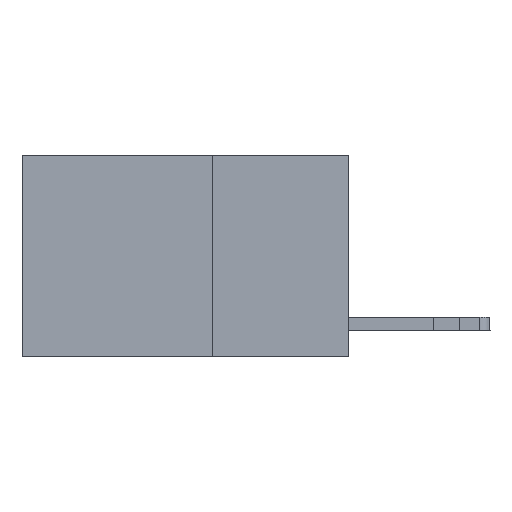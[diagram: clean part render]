
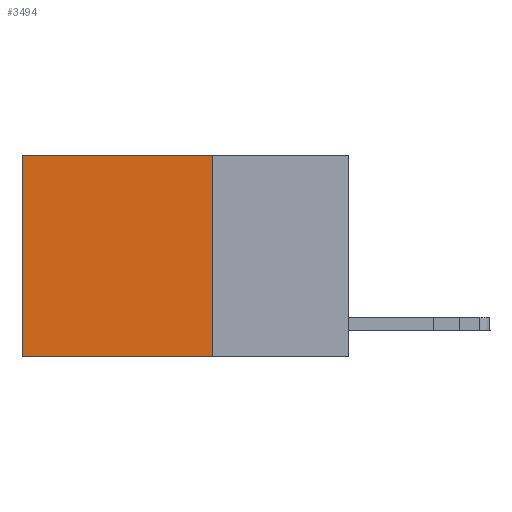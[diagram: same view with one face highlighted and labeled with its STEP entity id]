
A CAD part, left-side view. The second image highlights one B-rep face of the part: STEP entity #3494.
In plain terms, the highlighted planar face has unit normal (-1, 0, 0).
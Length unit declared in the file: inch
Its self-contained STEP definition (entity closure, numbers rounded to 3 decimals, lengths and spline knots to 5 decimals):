
#632 = ORIENTED_EDGE ( 'NONE', *, *, #12748, .T. ) ;
#1769 = VECTOR ( 'NONE', #14130, 39.37008 ) ;
#1792 = CARTESIAN_POINT ( 'NONE',  ( 0.2625, 0.25, 0. ) ) ;
#2085 = CARTESIAN_POINT ( 'NONE',  ( 0.2625, 0.25, -0.37 ) ) ;
#2788 = VECTOR ( 'NONE', #20159, 39.37008 ) ;
#2978 = VECTOR ( 'NONE', #10140, 39.37008 ) ;
#3494 = ADVANCED_FACE ( 'NONE', ( #3748 ), #18548, .F. ) ;
#3636 = LINE ( 'NONE', #5461, #2978 ) ;
#3684 = ORIENTED_EDGE ( 'NONE', *, *, #6785, .F. ) ;
#3748 = FACE_OUTER_BOUND ( 'NONE', #7550, .T. ) ;
#4170 = CARTESIAN_POINT ( 'NONE',  ( 0.2625, 0.6, 0. ) ) ;
#5211 = AXIS2_PLACEMENT_3D ( 'NONE', #11943, #18334, #7277 ) ;
#5420 = LINE ( 'NONE', #1792, #6610 ) ;
#5461 = CARTESIAN_POINT ( 'NONE',  ( 0.2625, 0.6, 0. ) ) ;
#5915 = CARTESIAN_POINT ( 'NONE',  ( 0.2625, 0.6, -0.37 ) ) ;
#6511 = ORIENTED_EDGE ( 'NONE', *, *, #18447, .T. ) ;
#6610 = VECTOR ( 'NONE', #11697, 39.37008 ) ;
#6785 = EDGE_CURVE ( 'NONE', #21086, #20830, #5420, .T. ) ;
#7277 = DIRECTION ( 'NONE',  ( 0., 0., -1. ) ) ;
#7550 = EDGE_LOOP ( 'NONE', ( #632, #9559, #3684, #6511 ) ) ;
#7853 = LINE ( 'NONE', #14338, #1769 ) ;
#9453 = VERTEX_POINT ( 'NONE', #4170 ) ;
#9559 = ORIENTED_EDGE ( 'NONE', *, *, #18653, .F. ) ;
#10140 = DIRECTION ( 'NONE',  ( 0., 0., -1. ) ) ;
#11697 = DIRECTION ( 'NONE',  ( 0., 0., -1. ) ) ;
#11943 = CARTESIAN_POINT ( 'NONE',  ( 0.2625, 0.25, 0. ) ) ;
#12748 = EDGE_CURVE ( 'NONE', #9453, #16873, #3636, .T. ) ;
#13754 = CARTESIAN_POINT ( 'NONE',  ( 0.2625, 0.25, -0.37 ) ) ;
#14130 = DIRECTION ( 'NONE',  ( 0., 1., 0. ) ) ;
#14338 = CARTESIAN_POINT ( 'NONE',  ( 0.2625, 0.25, 0. ) ) ;
#15462 = LINE ( 'NONE', #13754, #2788 ) ;
#16873 = VERTEX_POINT ( 'NONE', #5915 ) ;
#18334 = DIRECTION ( 'NONE',  ( 1., 0., 0. ) ) ;
#18447 = EDGE_CURVE ( 'NONE', #21086, #9453, #7853, .T. ) ;
#18548 = PLANE ( 'NONE',  #5211 ) ;
#18653 = EDGE_CURVE ( 'NONE', #20830, #16873, #15462, .T. ) ;
#19169 = CARTESIAN_POINT ( 'NONE',  ( 0.2625, 0.25, 0. ) ) ;
#20159 = DIRECTION ( 'NONE',  ( 0., 1., 0. ) ) ;
#20830 = VERTEX_POINT ( 'NONE', #2085 ) ;
#21086 = VERTEX_POINT ( 'NONE', #19169 ) ;
